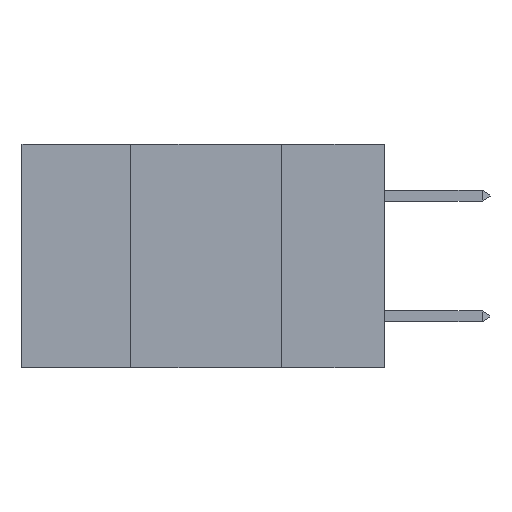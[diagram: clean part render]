
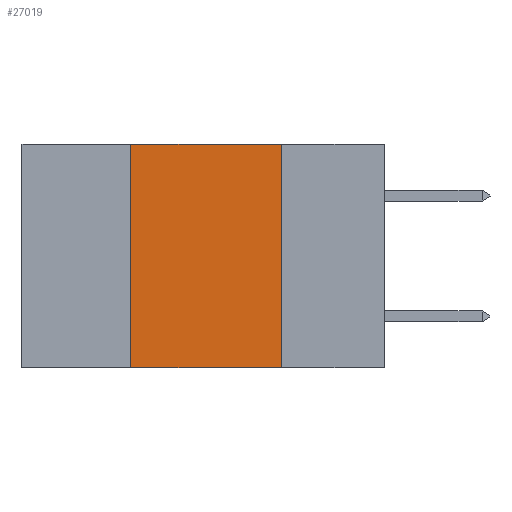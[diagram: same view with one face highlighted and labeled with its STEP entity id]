
A CAD part, left-side view. The second image highlights one B-rep face of the part: STEP entity #27019.
In plain terms, the highlighted planar face has unit normal (-1, 0, 0).
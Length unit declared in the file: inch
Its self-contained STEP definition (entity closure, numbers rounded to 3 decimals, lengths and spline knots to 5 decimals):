
#261 = LINE ( 'NONE', #396, #21444 ) ;
#290 = VERTEX_POINT ( 'NONE', #19061 ) ;
#396 = CARTESIAN_POINT ( 'NONE',  ( 0., 0.6, -0.37 ) ) ;
#846 = EDGE_CURVE ( 'NONE', #4255, #23898, #11391, .T. ) ;
#1411 = EDGE_LOOP ( 'NONE', ( #15786, #9994, #21818, #19726 ) ) ;
#1424 = PLANE ( 'NONE',  #12269 ) ;
#1536 = LINE ( 'NONE', #4285, #18649 ) ;
#2700 = DIRECTION ( 'NONE',  ( 0., 0., 1. ) ) ;
#3110 = CARTESIAN_POINT ( 'NONE',  ( 0., 0.42, 0. ) ) ;
#3175 = EDGE_CURVE ( 'NONE', #290, #23898, #261, .T. ) ;
#3726 = EDGE_CURVE ( 'NONE', #290, #26030, #19613, .T. ) ;
#4255 = VERTEX_POINT ( 'NONE', #23552 ) ;
#4285 = CARTESIAN_POINT ( 'NONE',  ( 0., 0.6, 0. ) ) ;
#5270 = VECTOR ( 'NONE', #2700, 39.37008 ) ;
#6778 = VECTOR ( 'NONE', #13568, 39.37008 ) ;
#7837 = DIRECTION ( 'NONE',  ( 0., -1., 0. ) ) ;
#9994 = ORIENTED_EDGE ( 'NONE', *, *, #20323, .F. ) ;
#10047 = DIRECTION ( 'NONE',  ( 1., 0., 0. ) ) ;
#11391 = LINE ( 'NONE', #19553, #6778 ) ;
#12237 = FACE_OUTER_BOUND ( 'NONE', #1411, .T. ) ;
#12269 = AXIS2_PLACEMENT_3D ( 'NONE', #20395, #10047, #24507 ) ;
#13568 = DIRECTION ( 'NONE',  ( 0., 0., -1. ) ) ;
#15786 = ORIENTED_EDGE ( 'NONE', *, *, #846, .F. ) ;
#17078 = CARTESIAN_POINT ( 'NONE',  ( 0., 0.17, -0.37 ) ) ;
#18649 = VECTOR ( 'NONE', #7837, 39.37008 ) ;
#19061 = CARTESIAN_POINT ( 'NONE',  ( 0., 0.42, -0.37 ) ) ;
#19553 = CARTESIAN_POINT ( 'NONE',  ( 0., 0.17, 0. ) ) ;
#19613 = LINE ( 'NONE', #3110, #5270 ) ;
#19726 = ORIENTED_EDGE ( 'NONE', *, *, #3175, .T. ) ;
#20323 = EDGE_CURVE ( 'NONE', #26030, #4255, #1536, .T. ) ;
#20395 = CARTESIAN_POINT ( 'NONE',  ( 0., 0.6, 0. ) ) ;
#20889 = DIRECTION ( 'NONE',  ( 0., -1., 0. ) ) ;
#21444 = VECTOR ( 'NONE', #20889, 39.37008 ) ;
#21818 = ORIENTED_EDGE ( 'NONE', *, *, #3726, .F. ) ;
#23484 = CARTESIAN_POINT ( 'NONE',  ( 0., 0.42, 0. ) ) ;
#23552 = CARTESIAN_POINT ( 'NONE',  ( 0., 0.17, 0. ) ) ;
#23898 = VERTEX_POINT ( 'NONE', #17078 ) ;
#24507 = DIRECTION ( 'NONE',  ( 0., 0., -1. ) ) ;
#26030 = VERTEX_POINT ( 'NONE', #23484 ) ;
#27019 = ADVANCED_FACE ( 'NONE', ( #12237 ), #1424, .F. ) ;
